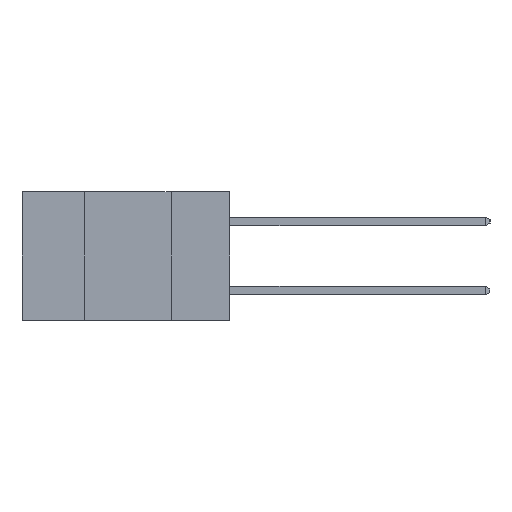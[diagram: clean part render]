
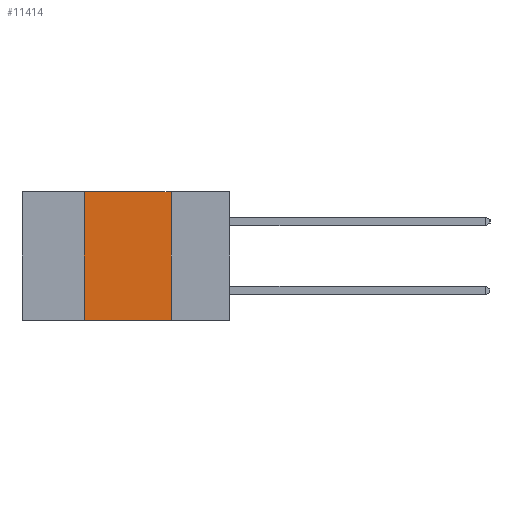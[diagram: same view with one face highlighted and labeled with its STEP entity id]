
A CAD part, left-side view. The second image highlights one B-rep face of the part: STEP entity #11414.
In plain terms, the highlighted planar face has unit normal (-1, 0, 0).
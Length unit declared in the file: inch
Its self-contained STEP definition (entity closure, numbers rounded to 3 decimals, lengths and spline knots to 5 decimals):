
#693 = PLANE ( 'NONE',  #12703 ) ;
#1199 = FACE_OUTER_BOUND ( 'NONE', #5334, .T. ) ;
#1425 = VERTEX_POINT ( 'NONE', #12780 ) ;
#1647 = EDGE_CURVE ( 'NONE', #14142, #7074, #12676, .T. ) ;
#1740 = EDGE_CURVE ( 'NONE', #7074, #13726, #8178, .T. ) ;
#1912 = CARTESIAN_POINT ( 'NONE',  ( 0., 0.17, 0. ) ) ;
#2130 = DIRECTION ( 'NONE',  ( 1., 0., 0. ) ) ;
#3251 = CARTESIAN_POINT ( 'NONE',  ( 0., 0.42, 0. ) ) ;
#3874 = VECTOR ( 'NONE', #11333, 39.37008 ) ;
#5160 = DIRECTION ( 'NONE',  ( 0., -1., 0. ) ) ;
#5233 = ORIENTED_EDGE ( 'NONE', *, *, #12465, .F. ) ;
#5334 = EDGE_LOOP ( 'NONE', ( #11847, #12283, #5233, #13137 ) ) ;
#5659 = CARTESIAN_POINT ( 'NONE',  ( 0., 0.42, 0. ) ) ;
#6298 = LINE ( 'NONE', #10938, #16985 ) ;
#7074 = VERTEX_POINT ( 'NONE', #17409 ) ;
#7151 = DIRECTION ( 'NONE',  ( 0., 0., 1. ) ) ;
#8178 = LINE ( 'NONE', #1912, #3874 ) ;
#9016 = VECTOR ( 'NONE', #5160, 39.37008 ) ;
#10584 = CARTESIAN_POINT ( 'NONE',  ( 0., 0.6, 0. ) ) ;
#10938 = CARTESIAN_POINT ( 'NONE',  ( 0., 0.6, -0.37 ) ) ;
#11148 = CARTESIAN_POINT ( 'NONE',  ( 0., 0.6, 0. ) ) ;
#11333 = DIRECTION ( 'NONE',  ( 0., 0., -1. ) ) ;
#11414 = ADVANCED_FACE ( 'NONE', ( #1199 ), #693, .F. ) ;
#11847 = ORIENTED_EDGE ( 'NONE', *, *, #1740, .F. ) ;
#11951 = CARTESIAN_POINT ( 'NONE',  ( 0., 0.17, -0.37 ) ) ;
#11977 = DIRECTION ( 'NONE',  ( 0., 0., -1. ) ) ;
#12283 = ORIENTED_EDGE ( 'NONE', *, *, #1647, .F. ) ;
#12465 = EDGE_CURVE ( 'NONE', #1425, #14142, #15971, .T. ) ;
#12676 = LINE ( 'NONE', #11148, #9016 ) ;
#12703 = AXIS2_PLACEMENT_3D ( 'NONE', #10584, #2130, #11977 ) ;
#12780 = CARTESIAN_POINT ( 'NONE',  ( 0., 0.42, -0.37 ) ) ;
#13028 = VECTOR ( 'NONE', #7151, 39.37008 ) ;
#13137 = ORIENTED_EDGE ( 'NONE', *, *, #15063, .T. ) ;
#13726 = VERTEX_POINT ( 'NONE', #11951 ) ;
#14142 = VERTEX_POINT ( 'NONE', #3251 ) ;
#15063 = EDGE_CURVE ( 'NONE', #1425, #13726, #6298, .T. ) ;
#15971 = LINE ( 'NONE', #5659, #13028 ) ;
#16186 = DIRECTION ( 'NONE',  ( 0., -1., 0. ) ) ;
#16985 = VECTOR ( 'NONE', #16186, 39.37008 ) ;
#17409 = CARTESIAN_POINT ( 'NONE',  ( 0., 0.17, 0. ) ) ;
